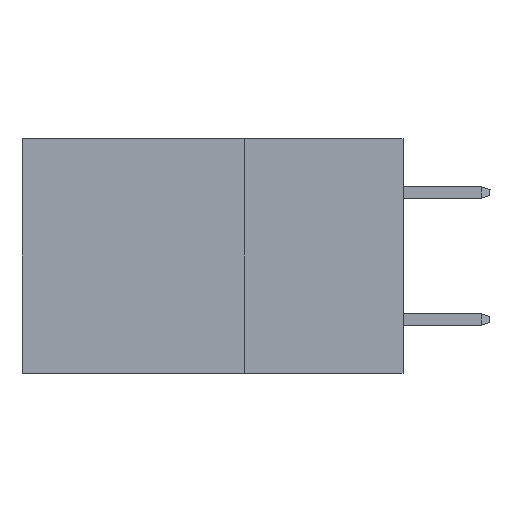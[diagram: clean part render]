
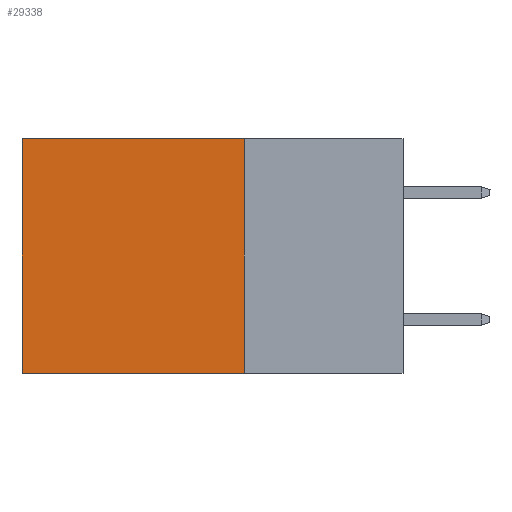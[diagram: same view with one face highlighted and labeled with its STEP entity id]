
A CAD part, left-side view. The second image highlights one B-rep face of the part: STEP entity #29338.
In plain terms, the highlighted planar face has unit normal (-1, 0, 0).
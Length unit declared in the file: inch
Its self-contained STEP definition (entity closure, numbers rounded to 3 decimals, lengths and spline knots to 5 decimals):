
#99 = VECTOR ( 'NONE', #15153, 39.37008 ) ;
#2199 = PLANE ( 'NONE',  #3151 ) ;
#3151 = AXIS2_PLACEMENT_3D ( 'NONE', #24611, #7511, #18723 ) ;
#3608 = VERTEX_POINT ( 'NONE', #29637 ) ;
#4450 = LINE ( 'NONE', #24657, #18886 ) ;
#4617 = ORIENTED_EDGE ( 'NONE', *, *, #16992, .T. ) ;
#5056 = ORIENTED_EDGE ( 'NONE', *, *, #16536, .T. ) ;
#6395 = VERTEX_POINT ( 'NONE', #35598 ) ;
#7240 = CARTESIAN_POINT ( 'NONE',  ( 0.2875, 0.25, -0.37 ) ) ;
#7511 = DIRECTION ( 'NONE',  ( 1., 0., 0. ) ) ;
#12397 = LINE ( 'NONE', #29131, #34170 ) ;
#12771 = DIRECTION ( 'NONE',  ( 0., 1., 0. ) ) ;
#14229 = ORIENTED_EDGE ( 'NONE', *, *, #17630, .F. ) ;
#15153 = DIRECTION ( 'NONE',  ( 0., 1., 0. ) ) ;
#15474 = LINE ( 'NONE', #18232, #19522 ) ;
#15518 = LINE ( 'NONE', #7240, #99 ) ;
#16445 = EDGE_CURVE ( 'NONE', #3608, #6395, #15518, .T. ) ;
#16536 = EDGE_CURVE ( 'NONE', #34320, #18067, #12397, .T. ) ;
#16992 = EDGE_CURVE ( 'NONE', #18067, #6395, #4450, .T. ) ;
#17630 = EDGE_CURVE ( 'NONE', #34320, #3608, #15474, .T. ) ;
#18067 = VERTEX_POINT ( 'NONE', #21282 ) ;
#18232 = CARTESIAN_POINT ( 'NONE',  ( 0.2875, 0.25, 0. ) ) ;
#18601 = DIRECTION ( 'NONE',  ( 0., 0., -1. ) ) ;
#18723 = DIRECTION ( 'NONE',  ( 0., 0., -1. ) ) ;
#18767 = ORIENTED_EDGE ( 'NONE', *, *, #16445, .F. ) ;
#18886 = VECTOR ( 'NONE', #21547, 39.37008 ) ;
#19522 = VECTOR ( 'NONE', #18601, 39.37008 ) ;
#21282 = CARTESIAN_POINT ( 'NONE',  ( 0.2875, 0.6, 0. ) ) ;
#21547 = DIRECTION ( 'NONE',  ( 0., 0., -1. ) ) ;
#24611 = CARTESIAN_POINT ( 'NONE',  ( 0.2875, 0.25, 0. ) ) ;
#24657 = CARTESIAN_POINT ( 'NONE',  ( 0.2875, 0.6, 0. ) ) ;
#27382 = FACE_OUTER_BOUND ( 'NONE', #28614, .T. ) ;
#28614 = EDGE_LOOP ( 'NONE', ( #4617, #18767, #14229, #5056 ) ) ;
#29131 = CARTESIAN_POINT ( 'NONE',  ( 0.2875, 0.25, 0. ) ) ;
#29338 = ADVANCED_FACE ( 'NONE', ( #27382 ), #2199, .F. ) ;
#29637 = CARTESIAN_POINT ( 'NONE',  ( 0.2875, 0.25, -0.37 ) ) ;
#34170 = VECTOR ( 'NONE', #12771, 39.37008 ) ;
#34320 = VERTEX_POINT ( 'NONE', #35680 ) ;
#35598 = CARTESIAN_POINT ( 'NONE',  ( 0.2875, 0.6, -0.37 ) ) ;
#35680 = CARTESIAN_POINT ( 'NONE',  ( 0.2875, 0.25, 0. ) ) ;
